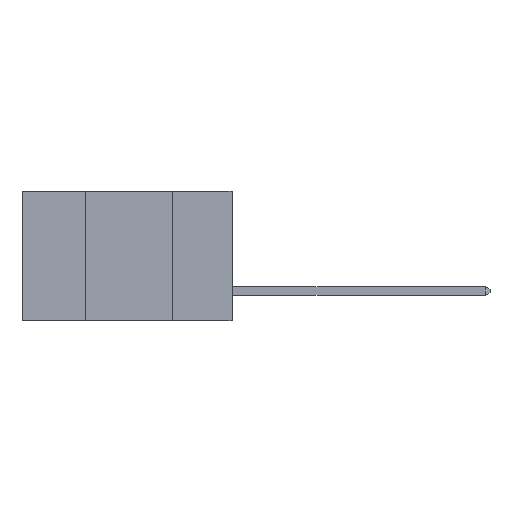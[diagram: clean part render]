
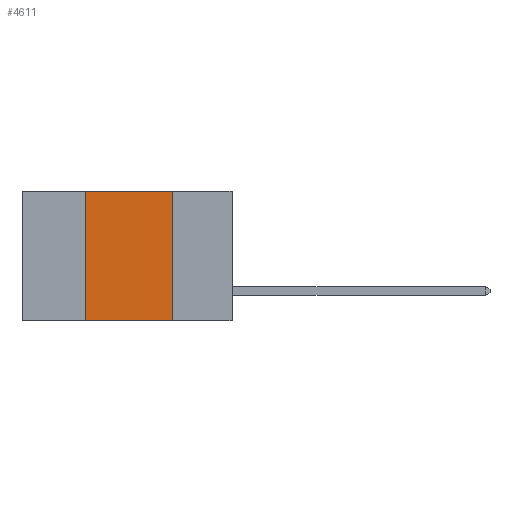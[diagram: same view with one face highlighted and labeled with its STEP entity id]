
A CAD part, left-side view. The second image highlights one B-rep face of the part: STEP entity #4611.
In plain terms, the highlighted planar face has unit normal (-1, 0, 0).
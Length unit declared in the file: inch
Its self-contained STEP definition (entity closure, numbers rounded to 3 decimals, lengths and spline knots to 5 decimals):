
#309 = ORIENTED_EDGE ( 'NONE', *, *, #6194, .F. ) ;
#338 = ORIENTED_EDGE ( 'NONE', *, *, #8892, .F. ) ;
#675 = VERTEX_POINT ( 'NONE', #12183 ) ;
#1475 = ORIENTED_EDGE ( 'NONE', *, *, #11955, .F. ) ;
#2127 = CARTESIAN_POINT ( 'NONE',  ( 0., 0.17, 0. ) ) ;
#3125 = CARTESIAN_POINT ( 'NONE',  ( 0., 0.42, -0.37 ) ) ;
#3225 = DIRECTION ( 'NONE',  ( 1., 0., 0. ) ) ;
#3232 = PLANE ( 'NONE',  #10084 ) ;
#3262 = CARTESIAN_POINT ( 'NONE',  ( 0., 0.6, 0. ) ) ;
#3334 = DIRECTION ( 'NONE',  ( 0., -1., 0. ) ) ;
#3642 = FACE_OUTER_BOUND ( 'NONE', #12695, .T. ) ;
#3762 = LINE ( 'NONE', #8135, #11828 ) ;
#3963 = VERTEX_POINT ( 'NONE', #4749 ) ;
#4611 = ADVANCED_FACE ( 'NONE', ( #3642 ), #3232, .F. ) ;
#4749 = CARTESIAN_POINT ( 'NONE',  ( 0., 0.17, -0.37 ) ) ;
#4804 = LINE ( 'NONE', #7196, #10257 ) ;
#5200 = VECTOR ( 'NONE', #3334, 39.37008 ) ;
#5566 = ORIENTED_EDGE ( 'NONE', *, *, #12974, .T. ) ;
#6194 = EDGE_CURVE ( 'NONE', #12571, #675, #3762, .T. ) ;
#6752 = CARTESIAN_POINT ( 'NONE',  ( 0., 0.6, 0. ) ) ;
#7196 = CARTESIAN_POINT ( 'NONE',  ( 0., 0.6, -0.37 ) ) ;
#7420 = LINE ( 'NONE', #6752, #5200 ) ;
#7764 = DIRECTION ( 'NONE',  ( 0., 0., -1. ) ) ;
#7826 = VERTEX_POINT ( 'NONE', #12916 ) ;
#8135 = CARTESIAN_POINT ( 'NONE',  ( 0., 0.42, 0. ) ) ;
#8252 = DIRECTION ( 'NONE',  ( 0., 0., -1. ) ) ;
#8255 = DIRECTION ( 'NONE',  ( 0., -1., 0. ) ) ;
#8864 = LINE ( 'NONE', #2127, #14151 ) ;
#8892 = EDGE_CURVE ( 'NONE', #7826, #3963, #8864, .T. ) ;
#9348 = DIRECTION ( 'NONE',  ( 0., 0., 1. ) ) ;
#10084 = AXIS2_PLACEMENT_3D ( 'NONE', #3262, #3225, #8252 ) ;
#10257 = VECTOR ( 'NONE', #8255, 39.37008 ) ;
#11828 = VECTOR ( 'NONE', #9348, 39.37008 ) ;
#11955 = EDGE_CURVE ( 'NONE', #675, #7826, #7420, .T. ) ;
#12183 = CARTESIAN_POINT ( 'NONE',  ( 0., 0.42, 0. ) ) ;
#12571 = VERTEX_POINT ( 'NONE', #3125 ) ;
#12695 = EDGE_LOOP ( 'NONE', ( #338, #1475, #309, #5566 ) ) ;
#12916 = CARTESIAN_POINT ( 'NONE',  ( 0., 0.17, 0. ) ) ;
#12974 = EDGE_CURVE ( 'NONE', #12571, #3963, #4804, .T. ) ;
#14151 = VECTOR ( 'NONE', #7764, 39.37008 ) ;
